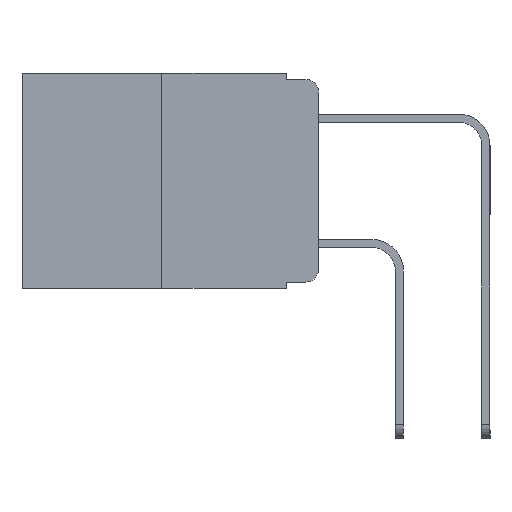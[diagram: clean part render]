
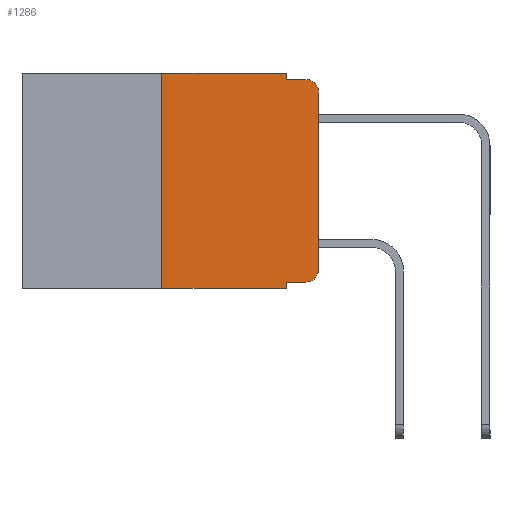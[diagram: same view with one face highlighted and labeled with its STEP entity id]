
A CAD part, left-side view. The second image highlights one B-rep face of the part: STEP entity #1286.
In plain terms, the highlighted planar face has unit normal (-1, 0, 0).
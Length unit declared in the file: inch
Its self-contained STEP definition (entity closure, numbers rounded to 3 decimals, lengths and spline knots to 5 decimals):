
#86 = VERTEX_POINT ( 'NONE', #16147 ) ;
#375 = ORIENTED_EDGE ( 'NONE', *, *, #14058, .T. ) ;
#421 = CARTESIAN_POINT ( 'NONE',  ( 0., 0.02, -0.333 ) ) ;
#653 = ORIENTED_EDGE ( 'NONE', *, *, #7952, .T. ) ;
#1286 = ADVANCED_FACE ( 'NONE', ( #14488 ), #11799, .F. ) ;
#1882 = VERTEX_POINT ( 'NONE', #10244 ) ;
#2068 = CARTESIAN_POINT ( 'NONE',  ( 0., 0.02, -0.03 ) ) ;
#2579 = CARTESIAN_POINT ( 'NONE',  ( 0., 0.051, 0. ) ) ;
#3562 = ORIENTED_EDGE ( 'NONE', *, *, #16987, .T. ) ;
#3581 = EDGE_CURVE ( 'NONE', #12532, #14164, #11090, .T. ) ;
#3736 = DIRECTION ( 'NONE',  ( 0., 0., -1. ) ) ;
#4130 = CARTESIAN_POINT ( 'NONE',  ( 0., 0., 0. ) ) ;
#4219 = VERTEX_POINT ( 'NONE', #16175 ) ;
#4488 = CARTESIAN_POINT ( 'NONE',  ( 0., 0.051, -0.333 ) ) ;
#5047 = VERTEX_POINT ( 'NONE', #421 ) ;
#5398 = VECTOR ( 'NONE', #8151, 39.37008 ) ;
#5418 = EDGE_LOOP ( 'NONE', ( #375, #6299, #15545, #10752, #19588, #17473, #9999, #16023, #3562, #653 ) ) ;
#5629 = AXIS2_PLACEMENT_3D ( 'NONE', #2068, #13589, #3736 ) ;
#5788 = LINE ( 'NONE', #4130, #14090 ) ;
#6108 = DIRECTION ( 'NONE',  ( 0., 0., -1. ) ) ;
#6117 = VECTOR ( 'NONE', #8861, 39.37008 ) ;
#6299 = ORIENTED_EDGE ( 'NONE', *, *, #8454, .T. ) ;
#6462 = EDGE_CURVE ( 'NONE', #1882, #18366, #18866, .T. ) ;
#6581 = CARTESIAN_POINT ( 'NONE',  ( 0., 0.051, -0.333 ) ) ;
#6760 = LINE ( 'NONE', #15923, #19550 ) ;
#7952 = EDGE_CURVE ( 'NONE', #5047, #8334, #17877, .T. ) ;
#8009 = LINE ( 'NONE', #2579, #17101 ) ;
#8151 = DIRECTION ( 'NONE',  ( 0., -1., 0. ) ) ;
#8334 = VERTEX_POINT ( 'NONE', #19916 ) ;
#8454 = EDGE_CURVE ( 'NONE', #86, #4219, #13235, .T. ) ;
#8715 = AXIS2_PLACEMENT_3D ( 'NONE', #19023, #9550, #20510 ) ;
#8861 = DIRECTION ( 'NONE',  ( 0., -1., 0. ) ) ;
#9060 = LINE ( 'NONE', #4488, #12921 ) ;
#9550 = DIRECTION ( 'NONE',  ( -1., 0., 0. ) ) ;
#9999 = ORIENTED_EDGE ( 'NONE', *, *, #3581, .T. ) ;
#10021 = VECTOR ( 'NONE', #20583, 39.37008 ) ;
#10244 = CARTESIAN_POINT ( 'NONE',  ( 0., 0.25, 0. ) ) ;
#10475 = VECTOR ( 'NONE', #19844, 39.37008 ) ;
#10525 = LINE ( 'NONE', #11264, #10021 ) ;
#10752 = ORIENTED_EDGE ( 'NONE', *, *, #19738, .F. ) ;
#11090 = LINE ( 'NONE', #14589, #6117 ) ;
#11264 = CARTESIAN_POINT ( 'NONE',  ( 0., 0.25, 0. ) ) ;
#11617 = EDGE_CURVE ( 'NONE', #19994, #14164, #8009, .T. ) ;
#11799 = PLANE ( 'NONE',  #20501 ) ;
#11903 = CARTESIAN_POINT ( 'NONE',  ( 0., 0.473, 0. ) ) ;
#12060 = DIRECTION ( 'NONE',  ( 1., 0., 0. ) ) ;
#12532 = VERTEX_POINT ( 'NONE', #14718 ) ;
#12633 = DIRECTION ( 'NONE',  ( 0., 0., -1. ) ) ;
#12640 = CARTESIAN_POINT ( 'NONE',  ( 0., 0.051, -0.343 ) ) ;
#12719 = DIRECTION ( 'NONE',  ( 0., -1., 0. ) ) ;
#12921 = VECTOR ( 'NONE', #12719, 39.37008 ) ;
#13235 = CIRCLE ( 'NONE', #5629, 0.02 ) ;
#13589 = DIRECTION ( 'NONE',  ( -1., 0., 0. ) ) ;
#14058 = EDGE_CURVE ( 'NONE', #8334, #86, #5788, .T. ) ;
#14076 = DIRECTION ( 'NONE',  ( 0., 0., -1. ) ) ;
#14090 = VECTOR ( 'NONE', #17104, 39.37008 ) ;
#14164 = VERTEX_POINT ( 'NONE', #12640 ) ;
#14488 = FACE_OUTER_BOUND ( 'NONE', #5418, .T. ) ;
#14589 = CARTESIAN_POINT ( 'NONE',  ( 0., 0.473, -0.343 ) ) ;
#14718 = CARTESIAN_POINT ( 'NONE',  ( 0., 0.25, -0.343 ) ) ;
#14861 = VERTEX_POINT ( 'NONE', #15157 ) ;
#15157 = CARTESIAN_POINT ( 'NONE',  ( 0., 0.051, -0.01 ) ) ;
#15545 = ORIENTED_EDGE ( 'NONE', *, *, #17136, .F. ) ;
#15923 = CARTESIAN_POINT ( 'NONE',  ( 0., 0.051, 0. ) ) ;
#16023 = ORIENTED_EDGE ( 'NONE', *, *, #11617, .F. ) ;
#16147 = CARTESIAN_POINT ( 'NONE',  ( 0., 0., -0.03 ) ) ;
#16155 = CARTESIAN_POINT ( 'NONE',  ( 0., 0.051, -0.01 ) ) ;
#16175 = CARTESIAN_POINT ( 'NONE',  ( 0., 0.02, -0.01 ) ) ;
#16579 = CARTESIAN_POINT ( 'NONE',  ( 0., 0.051, 0. ) ) ;
#16987 = EDGE_CURVE ( 'NONE', #19994, #5047, #9060, .T. ) ;
#17101 = VECTOR ( 'NONE', #14076, 39.37008 ) ;
#17104 = DIRECTION ( 'NONE',  ( 0., 0., 1. ) ) ;
#17136 = EDGE_CURVE ( 'NONE', #14861, #4219, #18290, .T. ) ;
#17473 = ORIENTED_EDGE ( 'NONE', *, *, #18625, .F. ) ;
#17877 = CIRCLE ( 'NONE', #8715, 0.02 ) ;
#18290 = LINE ( 'NONE', #16155, #5398 ) ;
#18366 = VERTEX_POINT ( 'NONE', #16579 ) ;
#18367 = CARTESIAN_POINT ( 'NONE',  ( 0., 0.473, 0. ) ) ;
#18625 = EDGE_CURVE ( 'NONE', #12532, #1882, #10525, .T. ) ;
#18866 = LINE ( 'NONE', #18367, #10475 ) ;
#19023 = CARTESIAN_POINT ( 'NONE',  ( 0., 0.02, -0.313 ) ) ;
#19550 = VECTOR ( 'NONE', #6108, 39.37008 ) ;
#19588 = ORIENTED_EDGE ( 'NONE', *, *, #6462, .F. ) ;
#19738 = EDGE_CURVE ( 'NONE', #18366, #14861, #6760, .T. ) ;
#19844 = DIRECTION ( 'NONE',  ( 0., -1., 0. ) ) ;
#19916 = CARTESIAN_POINT ( 'NONE',  ( 0., 0., -0.313 ) ) ;
#19994 = VERTEX_POINT ( 'NONE', #6581 ) ;
#20501 = AXIS2_PLACEMENT_3D ( 'NONE', #11903, #12060, #12633 ) ;
#20510 = DIRECTION ( 'NONE',  ( 0., 0., -1. ) ) ;
#20583 = DIRECTION ( 'NONE',  ( 0., 0., 1. ) ) ;
